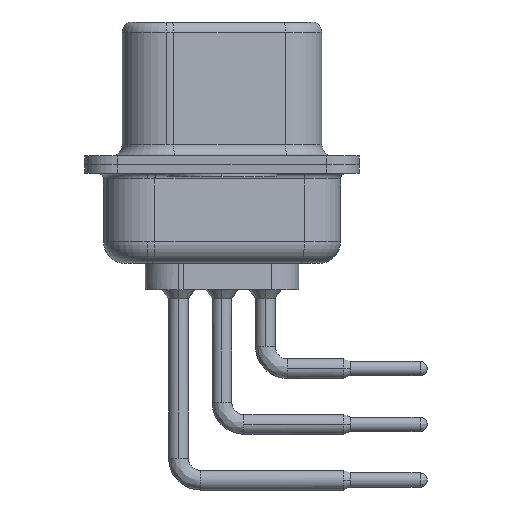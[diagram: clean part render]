
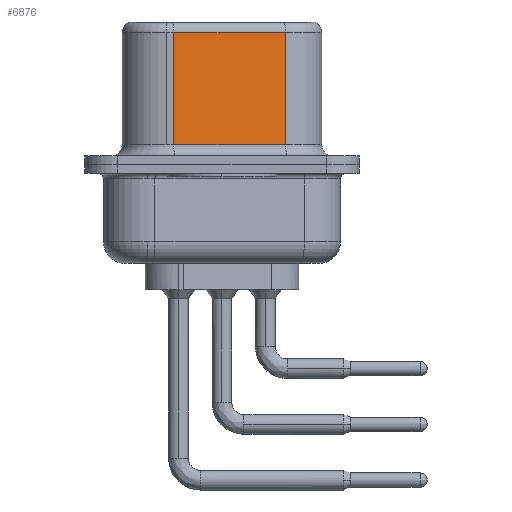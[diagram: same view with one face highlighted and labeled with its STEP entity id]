
A CAD part, left-side view. The second image highlights one B-rep face of the part: STEP entity #6876.
In plain terms, the highlighted planar face has unit normal (-0.985, -0.174, 0).
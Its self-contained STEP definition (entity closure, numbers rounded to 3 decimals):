
#60 = CARTESIAN_POINT ( 'NONE',  ( 4.555, -2.897, 6.02 ) ) ;
#158 = CARTESIAN_POINT ( 'NONE',  ( 4.555, -2.897, 0.9 ) ) ;
#418 = EDGE_CURVE ( 'NONE', #19177, #5816, #1450, .T. ) ;
#657 = ORIENTED_EDGE ( 'NONE', *, *, #418, .T. ) ;
#1174 = ORIENTED_EDGE ( 'NONE', *, *, #18389, .T. ) ;
#1450 = LINE ( 'NONE', #158, #22666 ) ;
#1547 = CARTESIAN_POINT ( 'NONE',  ( 3.655, 2.203, 6.52 ) ) ;
#2031 = VECTOR ( 'NONE', #22692, 1000. ) ;
#2530 = EDGE_CURVE ( 'NONE', #5206, #19177, #23845, .T. ) ;
#3579 = VECTOR ( 'NONE', #12732, 1000. ) ;
#3894 = FACE_OUTER_BOUND ( 'NONE', #15295, .T. ) ;
#4679 = ORIENTED_EDGE ( 'NONE', *, *, #25788, .F. ) ;
#4871 = CARTESIAN_POINT ( 'NONE',  ( 3.655, 2.203, 0.9 ) ) ;
#5206 = VERTEX_POINT ( 'NONE', #25847 ) ;
#5270 = DIRECTION ( 'NONE',  ( 0., 0., -1. ) ) ;
#5816 = VERTEX_POINT ( 'NONE', #12988 ) ;
#6691 = LINE ( 'NONE', #23525, #16912 ) ;
#6876 = ADVANCED_FACE ( 'NONE', ( #3894 ), #16959, .F. ) ;
#9785 = LINE ( 'NONE', #60, #3579 ) ;
#12732 = DIRECTION ( 'NONE',  ( -0.174, 0.985, 0. ) ) ;
#12988 = CARTESIAN_POINT ( 'NONE',  ( 4.555, -2.897, 0.9 ) ) ;
#14555 = AXIS2_PLACEMENT_3D ( 'NONE', #17099, #18845, #18720 ) ;
#15295 = EDGE_LOOP ( 'NONE', ( #4679, #1174, #22017, #657 ) ) ;
#16912 = VECTOR ( 'NONE', #5270, 1000. ) ;
#16959 = PLANE ( 'NONE',  #14555 ) ;
#17099 = CARTESIAN_POINT ( 'NONE',  ( 4.555, -2.897, 6.52 ) ) ;
#18389 = EDGE_CURVE ( 'NONE', #19498, #5206, #9785, .T. ) ;
#18720 = DIRECTION ( 'NONE',  ( -0.174, 0.985, 0. ) ) ;
#18845 = DIRECTION ( 'NONE',  ( 0.985, 0.174, 0. ) ) ;
#19177 = VERTEX_POINT ( 'NONE', #4871 ) ;
#19498 = VERTEX_POINT ( 'NONE', #26557 ) ;
#22017 = ORIENTED_EDGE ( 'NONE', *, *, #2530, .T. ) ;
#22666 = VECTOR ( 'NONE', #24692, 1000. ) ;
#22692 = DIRECTION ( 'NONE',  ( 0., 0., -1. ) ) ;
#23525 = CARTESIAN_POINT ( 'NONE',  ( 4.555, -2.897, 6.52 ) ) ;
#23845 = LINE ( 'NONE', #1547, #2031 ) ;
#24692 = DIRECTION ( 'NONE',  ( 0.174, -0.985, 0. ) ) ;
#25788 = EDGE_CURVE ( 'NONE', #19498, #5816, #6691, .T. ) ;
#25847 = CARTESIAN_POINT ( 'NONE',  ( 3.655, 2.203, 6.02 ) ) ;
#26557 = CARTESIAN_POINT ( 'NONE',  ( 4.555, -2.897, 6.02 ) ) ;
